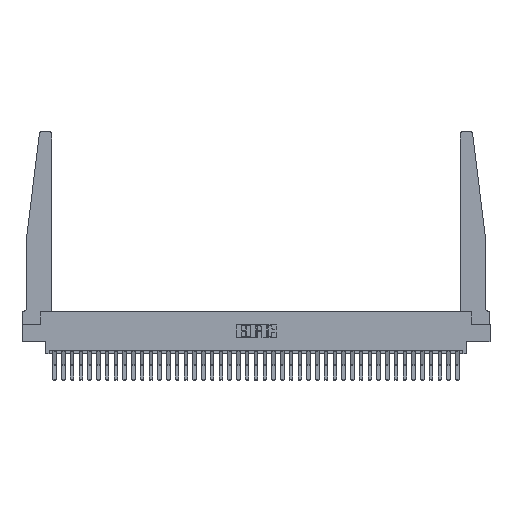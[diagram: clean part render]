
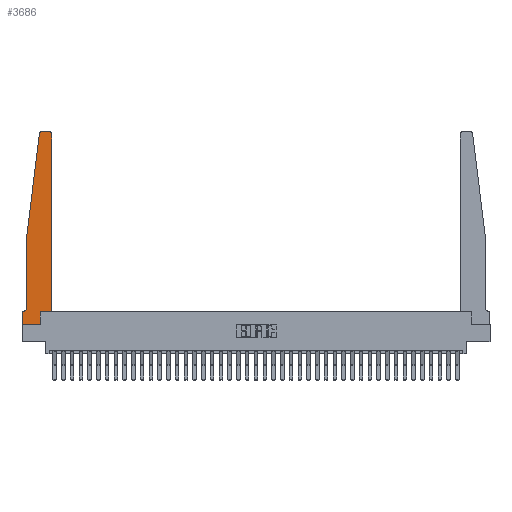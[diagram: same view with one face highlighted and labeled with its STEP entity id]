
A CAD part, top view. The second image highlights one B-rep face of the part: STEP entity #3686.
In plain terms, the highlighted planar face has unit normal (0, 0, 1).
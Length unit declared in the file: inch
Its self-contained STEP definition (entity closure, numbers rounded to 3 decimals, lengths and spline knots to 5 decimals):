
#56 = ORIENTED_EDGE ( 'NONE', *, *, #13523, .T. ) ;
#200 = CIRCLE ( 'NONE', #31777, 0.03 ) ;
#247 = VERTEX_POINT ( 'NONE', #17561 ) ;
#488 = CARTESIAN_POINT ( 'NONE',  ( 0.065, 0.2375, 0.37 ) ) ;
#723 = CARTESIAN_POINT ( 'NONE',  ( 0.395, 2.72, 0.37 ) ) ;
#758 = CARTESIAN_POINT ( 'NONE',  ( 0.425, 0.18, 0.37 ) ) ;
#837 = DIRECTION ( 'NONE',  ( -1., 0., 0. ) ) ;
#945 = DIRECTION ( 'NONE',  ( 0., 1., 0. ) ) ;
#1244 = CARTESIAN_POINT ( 'NONE',  ( 0.395, 2.75, 0.37 ) ) ;
#1579 = EDGE_LOOP ( 'NONE', ( #33500, #23311, #7246, #24600, #26678, #32167, #56, #16895, #15162, #16856, #14691, #5849 ) ) ;
#1581 = VERTEX_POINT ( 'NONE', #28822 ) ;
#3340 = EDGE_CURVE ( 'NONE', #24292, #26373, #17792, .T. ) ;
#3451 = DIRECTION ( 'NONE',  ( 1., 0., 0. ) ) ;
#3686 = ADVANCED_FACE ( 'NONE', ( #6801 ), #20340, .T. ) ;
#4091 = CIRCLE ( 'NONE', #22573, 0.03 ) ;
#4428 = CARTESIAN_POINT ( 'NONE',  ( 0.2605, 0., 0.37 ) ) ;
#4755 = DIRECTION ( 'NONE',  ( 0., 1., 0. ) ) ;
#4991 = CARTESIAN_POINT ( 'NONE',  ( 0.27653, 2.75, 0.37 ) ) ;
#5025 = VERTEX_POINT ( 'NONE', #4428 ) ;
#5723 = CARTESIAN_POINT ( 'NONE',  ( 0.065, 0.1875, 0.37 ) ) ;
#5737 = DIRECTION ( 'NONE',  ( 1., 0., 0. ) ) ;
#5849 = ORIENTED_EDGE ( 'NONE', *, *, #15524, .T. ) ;
#6014 = EDGE_CURVE ( 'NONE', #247, #24292, #17665, .T. ) ;
#6372 = EDGE_CURVE ( 'NONE', #5025, #24391, #12963, .T. ) ;
#6801 = FACE_OUTER_BOUND ( 'NONE', #1579, .T. ) ;
#6828 = EDGE_CURVE ( 'NONE', #19695, #5025, #11864, .T. ) ;
#6862 = CARTESIAN_POINT ( 'NONE',  ( 0.015, 0.2375, 0.37 ) ) ;
#7246 = ORIENTED_EDGE ( 'NONE', *, *, #6014, .T. ) ;
#8105 = DIRECTION ( 'NONE',  ( 0., 0., 1. ) ) ;
#9429 = CARTESIAN_POINT ( 'NONE',  ( 0.2605, 0.18, 0.37 ) ) ;
#9498 = VECTOR ( 'NONE', #16904, 39.37008 ) ;
#9585 = DIRECTION ( 'NONE',  ( -1., 0., 0. ) ) ;
#10018 = CARTESIAN_POINT ( 'NONE',  ( 0.425, 0.18, 0.37 ) ) ;
#10399 = LINE ( 'NONE', #33197, #31101 ) ;
#10789 = CARTESIAN_POINT ( 'NONE',  ( 0.065, 1.25, 0.37 ) ) ;
#11037 = VECTOR ( 'NONE', #5737, 39.37008 ) ;
#11553 = EDGE_CURVE ( 'NONE', #14175, #247, #200, .T. ) ;
#11864 = LINE ( 'NONE', #19184, #11037 ) ;
#12118 = EDGE_CURVE ( 'NONE', #18413, #1581, #19155, .T. ) ;
#12278 = CARTESIAN_POINT ( 'NONE',  ( 0., 0.1875, 0.37 ) ) ;
#12818 = DIRECTION ( 'NONE',  ( -0.122, -0.992, 0. ) ) ;
#12963 = LINE ( 'NONE', #14345, #21027 ) ;
#13480 = DIRECTION ( 'NONE',  ( 0., -1., 0. ) ) ;
#13523 = EDGE_CURVE ( 'NONE', #14027, #19695, #29135, .T. ) ;
#14027 = VERTEX_POINT ( 'NONE', #34177 ) ;
#14175 = VERTEX_POINT ( 'NONE', #4991 ) ;
#14230 = CARTESIAN_POINT ( 'NONE',  ( 0.065, 1.25, 0.37 ) ) ;
#14345 = CARTESIAN_POINT ( 'NONE',  ( 0.2605, 0.18, 0.37 ) ) ;
#14691 = ORIENTED_EDGE ( 'NONE', *, *, #12118, .T. ) ;
#14921 = LINE ( 'NONE', #758, #9498 ) ;
#15162 = ORIENTED_EDGE ( 'NONE', *, *, #6372, .T. ) ;
#15524 = EDGE_CURVE ( 'NONE', #1581, #27164, #4091, .T. ) ;
#15568 = VECTOR ( 'NONE', #19170, 39.37008 ) ;
#15581 = EDGE_CURVE ( 'NONE', #27164, #14175, #10399, .T. ) ;
#16856 = ORIENTED_EDGE ( 'NONE', *, *, #22085, .T. ) ;
#16895 = ORIENTED_EDGE ( 'NONE', *, *, #6828, .T. ) ;
#16904 = DIRECTION ( 'NONE',  ( 1., 0., 0. ) ) ;
#17056 = CIRCLE ( 'NONE', #32318, 0.05 ) ;
#17561 = CARTESIAN_POINT ( 'NONE',  ( 0.24675, 2.72367, 0.37 ) ) ;
#17665 = LINE ( 'NONE', #34491, #24040 ) ;
#17724 = DIRECTION ( 'NONE',  ( 1., 0., 0. ) ) ;
#17792 = LINE ( 'NONE', #10789, #19511 ) ;
#18413 = VERTEX_POINT ( 'NONE', #10018 ) ;
#19155 = LINE ( 'NONE', #28927, #24670 ) ;
#19170 = DIRECTION ( 'NONE',  ( -1., 0., 0. ) ) ;
#19184 = CARTESIAN_POINT ( 'NONE',  ( 0., 0., 0.37 ) ) ;
#19511 = VECTOR ( 'NONE', #13480, 39.37008 ) ;
#19590 = DIRECTION ( 'NONE',  ( 0., 0., 1. ) ) ;
#19695 = VERTEX_POINT ( 'NONE', #20913 ) ;
#20340 = PLANE ( 'NONE',  #31600 ) ;
#20913 = CARTESIAN_POINT ( 'NONE',  ( 0., 0., 0.37 ) ) ;
#21027 = VECTOR ( 'NONE', #945, 39.37008 ) ;
#22085 = EDGE_CURVE ( 'NONE', #24391, #18413, #14921, .T. ) ;
#22266 = EDGE_CURVE ( 'NONE', #26373, #26471, #17056, .T. ) ;
#22573 = AXIS2_PLACEMENT_3D ( 'NONE', #723, #19590, #3451 ) ;
#23311 = ORIENTED_EDGE ( 'NONE', *, *, #11553, .T. ) ;
#24040 = VECTOR ( 'NONE', #12818, 39.37008 ) ;
#24185 = CARTESIAN_POINT ( 'NONE',  ( 0., 0., 0.37 ) ) ;
#24284 = CARTESIAN_POINT ( 'NONE',  ( 0.27653, 2.72, 0.37 ) ) ;
#24292 = VERTEX_POINT ( 'NONE', #14230 ) ;
#24391 = VERTEX_POINT ( 'NONE', #9429 ) ;
#24600 = ORIENTED_EDGE ( 'NONE', *, *, #3340, .T. ) ;
#24670 = VECTOR ( 'NONE', #4755, 39.37008 ) ;
#25767 = DIRECTION ( 'NONE',  ( 0., 0., -1. ) ) ;
#26373 = VERTEX_POINT ( 'NONE', #488 ) ;
#26471 = VERTEX_POINT ( 'NONE', #30546 ) ;
#26678 = ORIENTED_EDGE ( 'NONE', *, *, #22266, .T. ) ;
#26987 = DIRECTION ( 'NONE',  ( 1., 0., 0. ) ) ;
#26993 = DIRECTION ( 'NONE',  ( 0., -1., 0. ) ) ;
#27164 = VERTEX_POINT ( 'NONE', #1244 ) ;
#28822 = CARTESIAN_POINT ( 'NONE',  ( 0.425, 2.72, 0.37 ) ) ;
#28927 = CARTESIAN_POINT ( 'NONE',  ( 0.425, 0.18, 0.37 ) ) ;
#29135 = LINE ( 'NONE', #24185, #30839 ) ;
#30546 = CARTESIAN_POINT ( 'NONE',  ( 0.015, 0.1875, 0.37 ) ) ;
#30811 = LINE ( 'NONE', #5723, #15568 ) ;
#30839 = VECTOR ( 'NONE', #26993, 39.37008 ) ;
#31018 = EDGE_CURVE ( 'NONE', #26471, #14027, #30811, .T. ) ;
#31101 = VECTOR ( 'NONE', #837, 39.37008 ) ;
#31600 = AXIS2_PLACEMENT_3D ( 'NONE', #12278, #33938, #17724 ) ;
#31777 = AXIS2_PLACEMENT_3D ( 'NONE', #24284, #8105, #26987 ) ;
#32167 = ORIENTED_EDGE ( 'NONE', *, *, #31018, .T. ) ;
#32318 = AXIS2_PLACEMENT_3D ( 'NONE', #6862, #25767, #9585 ) ;
#33197 = CARTESIAN_POINT ( 'NONE',  ( 0.25, 2.75, 0.37 ) ) ;
#33500 = ORIENTED_EDGE ( 'NONE', *, *, #15581, .T. ) ;
#33938 = DIRECTION ( 'NONE',  ( 0., 0., 1. ) ) ;
#34177 = CARTESIAN_POINT ( 'NONE',  ( 0., 0.1875, 0.37 ) ) ;
#34491 = CARTESIAN_POINT ( 'NONE',  ( 0.065, 1.25, 0.37 ) ) ;
